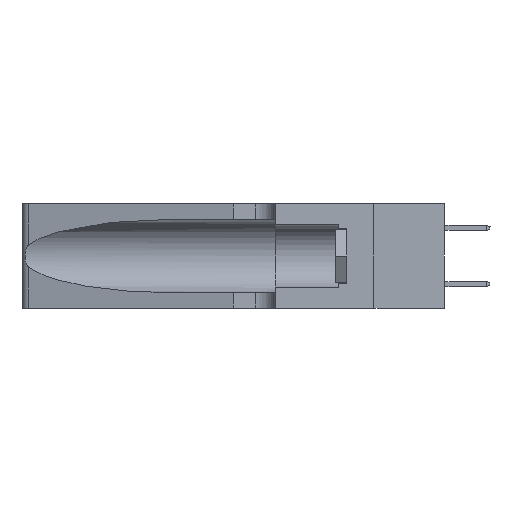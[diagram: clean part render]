
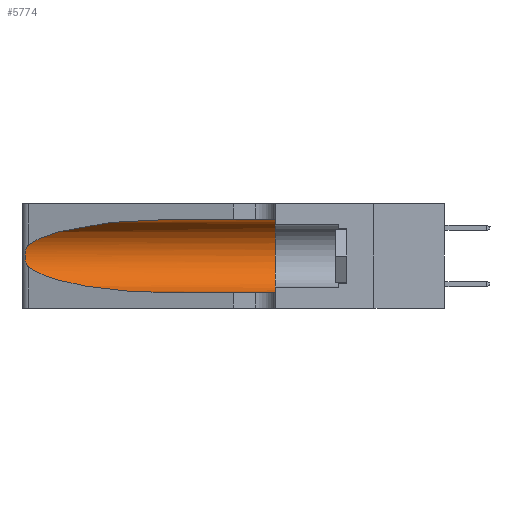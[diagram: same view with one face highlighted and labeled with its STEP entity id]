
A CAD part, left-side view. The second image highlights one B-rep face of the part: STEP entity #5774.
In plain terms, the highlighted cylindrical face has radius 3.308 mm (diameter 6.617 mm), a partial arc.
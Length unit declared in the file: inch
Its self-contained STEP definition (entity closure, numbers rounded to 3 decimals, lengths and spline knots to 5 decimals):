
#380 = CARTESIAN_POINT ( 'NONE',  ( 0.1305, 1.61858, 0.31525 ) ) ;
#457 = CARTESIAN_POINT ( 'NONE',  ( 0.25789, 1.23486, 0.15765 ) ) ;
#592 = B_SPLINE_CURVE_WITH_KNOTS ( 'NONE', 3,
 ( #2493, #14988, #19075, #6783, #21133, #8903, #23147, #10966, #25205, #13026, #457, #15073, #2590, #17101 ),
 .UNSPECIFIED., .F., .F.,
 ( 4, 2, 2, 2, 2, 2, 4 ),
 ( 0., 0.00027, 0.00053, 0.00107, 0.0016, 0.00187, 0.00214 ),
 .UNSPECIFIED. ) ;
#687 = CARTESIAN_POINT ( 'NONE',  ( 0.25487, 1.22718, 0.14631 ) ) ;
#840 = EDGE_CURVE ( 'NONE', #19776, #2390, #12388, .T. ) ;
#1077 = VERTEX_POINT ( 'NONE', #11587 ) ;
#1165 = VERTEX_POINT ( 'NONE', #25228 ) ;
#1738 = CARTESIAN_POINT ( 'NONE',  ( 0.1305, 0.72297, 0.31525 ) ) ;
#2000 = VERTEX_POINT ( 'NONE', #20746 ) ;
#2390 = VERTEX_POINT ( 'NONE', #24604 ) ;
#2493 = CARTESIAN_POINT ( 'NONE',  ( 0.25487, 1.22718, 0.22369 ) ) ;
#2590 = CARTESIAN_POINT ( 'NONE',  ( 0.25555, 1.22993, 0.14849 ) ) ;
#3478 = DIRECTION ( 'NONE',  ( 0., 1., 0. ) ) ;
#3554 = VECTOR ( 'NONE', #8256, 39.37008 ) ;
#3863 = CARTESIAN_POINT ( 'NONE',  ( 0.2373, 1.15595, 0.28018 ) ) ;
#3943 = EDGE_CURVE ( 'NONE', #1165, #22226, #24615, .T. ) ;
#4778 = EDGE_CURVE ( 'NONE', #2390, #1077, #18538, .T. ) ;
#5567 = ORIENTED_EDGE ( 'NONE', *, *, #3943, .T. ) ;
#5774 = ADVANCED_FACE ( 'NONE', ( #7911 ), #23572, .F. ) ;
#6124 = CARTESIAN_POINT ( 'NONE',  ( 0.1305, 1.61858, 0.05475 ) ) ;
#6783 = CARTESIAN_POINT ( 'NONE',  ( 0.25787, 1.23484, 0.2124 ) ) ;
#6811 = DIRECTION ( 'NONE',  ( 0., 0., -1. ) ) ;
#6879 = EDGE_CURVE ( 'NONE', #22226, #1077, #24841, .T. ) ;
#6883 = VECTOR ( 'NONE', #24771, 39.37008 ) ;
#7094 = CARTESIAN_POINT ( 'NONE',  ( 0.1305, 0.72297, 0.05475 ) ) ;
#7911 = FACE_OUTER_BOUND ( 'NONE', #26691, .T. ) ;
#8256 = DIRECTION ( 'NONE',  ( 0., -1., 0. ) ) ;
#8307 = AXIS2_PLACEMENT_3D ( 'NONE', #15942, #3478, #17952 ) ;
#8903 = CARTESIAN_POINT ( 'NONE',  ( 0.26018, 1.23835, 0.19895 ) ) ;
#8934 = CARTESIAN_POINT ( 'NONE',  ( 0.2373, 1.15595, 0.08982 ) ) ;
#9055 = CARTESIAN_POINT ( 'NONE',  ( 0.1305, 0.72297, 0.05475 ) ) ;
#10920 = AXIS2_PLACEMENT_3D ( 'NONE', #19103, #17042, #6811 ) ;
#10966 = CARTESIAN_POINT ( 'NONE',  ( 0.26075, 1.23896, 0.178 ) ) ;
#11587 = CARTESIAN_POINT ( 'NONE',  ( 0.1305, 0.35, 0.05475 ) ) ;
#12378 = EDGE_CURVE ( 'NONE', #2000, #1165, #592, .T. ) ;
#12388 = LINE ( 'NONE', #380, #6883 ) ;
#13026 = CARTESIAN_POINT ( 'NONE',  ( 0.25856, 1.23593, 0.16098 ) ) ;
#14694 = ORIENTED_EDGE ( 'NONE', *, *, #6879, .T. ) ;
#14988 = CARTESIAN_POINT ( 'NONE',  ( 0.25555, 1.22994, 0.2215 ) ) ;
#15073 = CARTESIAN_POINT ( 'NONE',  ( 0.25639, 1.23186, 0.15144 ) ) ;
#15942 = CARTESIAN_POINT ( 'NONE',  ( 0.1305, 0.35, 0.185 ) ) ;
#16010 = ORIENTED_EDGE ( 'NONE', *, *, #12378, .T. ) ;
#16891 = EDGE_CURVE ( 'NONE', #19776, #2000, #17889, .T. ) ;
#17024 = ORIENTED_EDGE ( 'NONE', *, *, #840, .F. ) ;
#17042 = DIRECTION ( 'NONE',  ( 0., -1., 0. ) ) ;
#17101 = CARTESIAN_POINT ( 'NONE',  ( 0.25487, 1.22718, 0.14631 ) ) ;
#17889 =( BOUNDED_CURVE ( )  B_SPLINE_CURVE ( 3, ( #1738, #26444, #3863, #18334 ),
 .UNSPECIFIED., .F., .F. ) 
 B_SPLINE_CURVE_WITH_KNOTS ( ( 4, 4 ),
 ( 1.5708, 2.84003 ),
 .UNSPECIFIED. ) 
 CURVE ( )  GEOMETRIC_REPRESENTATION_ITEM ( )  RATIONAL_B_SPLINE_CURVE ( ( 1., 0.87, 0.87, 1. ) ) 
 REPRESENTATION_ITEM ( '' )  );
#17952 = DIRECTION ( 'NONE',  ( 0., 0., 1. ) ) ;
#18334 = CARTESIAN_POINT ( 'NONE',  ( 0.25487, 1.22718, 0.22369 ) ) ;
#18538 = CIRCLE ( 'NONE', #8307, 0.13025 ) ;
#18627 = CARTESIAN_POINT ( 'NONE',  ( 0.1305, 0.72297, 0.31525 ) ) ;
#19075 = CARTESIAN_POINT ( 'NONE',  ( 0.25639, 1.23184, 0.21858 ) ) ;
#19103 = CARTESIAN_POINT ( 'NONE',  ( 0.1305, 1.61858, 0.185 ) ) ;
#19379 = CARTESIAN_POINT ( 'NONE',  ( 0.18966, 0.96281, 0.05475 ) ) ;
#19776 = VERTEX_POINT ( 'NONE', #18627 ) ;
#20746 = CARTESIAN_POINT ( 'NONE',  ( 0.25487, 1.22718, 0.22369 ) ) ;
#21133 = CARTESIAN_POINT ( 'NONE',  ( 0.25854, 1.2359, 0.20912 ) ) ;
#22226 = VERTEX_POINT ( 'NONE', #9055 ) ;
#23147 = CARTESIAN_POINT ( 'NONE',  ( 0.26075, 1.23896, 0.19203 ) ) ;
#23572 = CYLINDRICAL_SURFACE ( 'NONE', #10920, 0.13025 ) ;
#23643 = ORIENTED_EDGE ( 'NONE', *, *, #4778, .F. ) ;
#24604 = CARTESIAN_POINT ( 'NONE',  ( 0.1305, 0.35, 0.31525 ) ) ;
#24615 =( BOUNDED_CURVE ( )  B_SPLINE_CURVE ( 3, ( #687, #8934, #19379, #7094 ),
 .UNSPECIFIED., .F., .T. ) 
 B_SPLINE_CURVE_WITH_KNOTS ( ( 4, 4 ),
 ( 3.44316, 4.71239 ),
 .UNSPECIFIED. ) 
 CURVE ( )  GEOMETRIC_REPRESENTATION_ITEM ( )  RATIONAL_B_SPLINE_CURVE ( ( 1., 0.87, 0.87, 1. ) ) 
 REPRESENTATION_ITEM ( '' )  );
#24771 = DIRECTION ( 'NONE',  ( 0., -1., 0. ) ) ;
#24841 = LINE ( 'NONE', #6124, #3554 ) ;
#25205 = CARTESIAN_POINT ( 'NONE',  ( 0.26017, 1.23833, 0.17102 ) ) ;
#25228 = CARTESIAN_POINT ( 'NONE',  ( 0.25487, 1.22718, 0.14631 ) ) ;
#25381 = ORIENTED_EDGE ( 'NONE', *, *, #16891, .T. ) ;
#26444 = CARTESIAN_POINT ( 'NONE',  ( 0.18966, 0.96281, 0.31525 ) ) ;
#26691 = EDGE_LOOP ( 'NONE', ( #25381, #16010, #5567, #14694, #23643, #17024 ) ) ;
